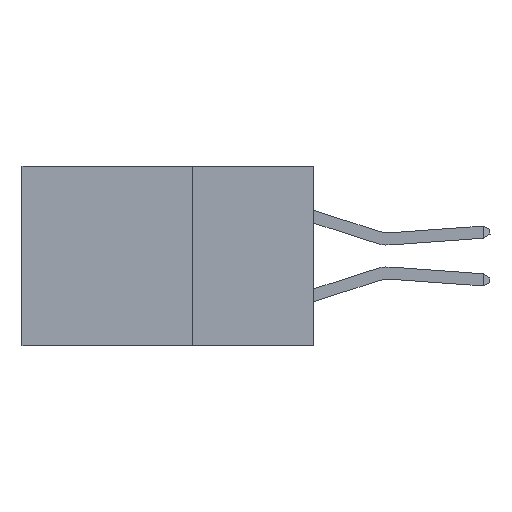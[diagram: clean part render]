
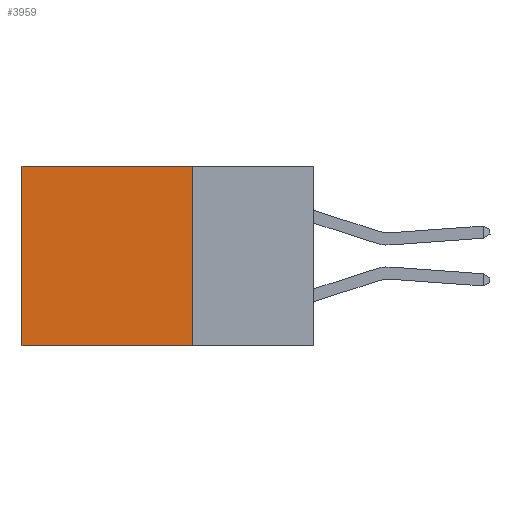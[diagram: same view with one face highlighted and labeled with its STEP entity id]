
A CAD part, left-side view. The second image highlights one B-rep face of the part: STEP entity #3959.
In plain terms, the highlighted planar face has unit normal (-1, 0, 0).
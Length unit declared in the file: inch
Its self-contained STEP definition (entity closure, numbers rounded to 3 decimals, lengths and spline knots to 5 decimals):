
#386 = CARTESIAN_POINT ( 'NONE',  ( 0.2875, 0.25, 0. ) ) ;
#739 = DIRECTION ( 'NONE',  ( 0., 1., 0. ) ) ;
#1558 = DIRECTION ( 'NONE',  ( 0., 0., -1. ) ) ;
#3090 = VECTOR ( 'NONE', #1558, 39.37008 ) ;
#3364 = PLANE ( 'NONE',  #15219 ) ;
#3959 = ADVANCED_FACE ( 'NONE', ( #17140 ), #3364, .F. ) ;
#4529 = CARTESIAN_POINT ( 'NONE',  ( 0.2875, 0.25, 0. ) ) ;
#6988 = ORIENTED_EDGE ( 'NONE', *, *, #11233, .T. ) ;
#7425 = CARTESIAN_POINT ( 'NONE',  ( 0.2875, 0.6, 0. ) ) ;
#7578 = LINE ( 'NONE', #13091, #13519 ) ;
#7761 = DIRECTION ( 'NONE',  ( 0., 0., -1. ) ) ;
#8370 = EDGE_LOOP ( 'NONE', ( #14749, #17801, #16557, #6988 ) ) ;
#8456 = LINE ( 'NONE', #4529, #12977 ) ;
#9046 = CARTESIAN_POINT ( 'NONE',  ( 0.2875, 0.25, -0.37 ) ) ;
#9297 = EDGE_CURVE ( 'NONE', #17252, #10705, #7578, .T. ) ;
#9495 = EDGE_CURVE ( 'NONE', #17716, #13127, #11349, .T. ) ;
#10125 = EDGE_CURVE ( 'NONE', #13127, #10705, #14400, .T. ) ;
#10705 = VERTEX_POINT ( 'NONE', #15139 ) ;
#11233 = EDGE_CURVE ( 'NONE', #17716, #17252, #8456, .T. ) ;
#11349 = LINE ( 'NONE', #14056, #3090 ) ;
#11608 = CARTESIAN_POINT ( 'NONE',  ( 0.2875, 0.25, -0.37 ) ) ;
#12096 = VECTOR ( 'NONE', #739, 39.37008 ) ;
#12977 = VECTOR ( 'NONE', #15205, 39.37008 ) ;
#13091 = CARTESIAN_POINT ( 'NONE',  ( 0.2875, 0.6, 0. ) ) ;
#13127 = VERTEX_POINT ( 'NONE', #9046 ) ;
#13519 = VECTOR ( 'NONE', #7761, 39.37008 ) ;
#14051 = DIRECTION ( 'NONE',  ( 0., 0., -1. ) ) ;
#14056 = CARTESIAN_POINT ( 'NONE',  ( 0.2875, 0.25, 0. ) ) ;
#14321 = DIRECTION ( 'NONE',  ( 1., 0., 0. ) ) ;
#14400 = LINE ( 'NONE', #11608, #12096 ) ;
#14749 = ORIENTED_EDGE ( 'NONE', *, *, #9297, .T. ) ;
#14881 = CARTESIAN_POINT ( 'NONE',  ( 0.2875, 0.25, 0. ) ) ;
#15139 = CARTESIAN_POINT ( 'NONE',  ( 0.2875, 0.6, -0.37 ) ) ;
#15205 = DIRECTION ( 'NONE',  ( 0., 1., 0. ) ) ;
#15219 = AXIS2_PLACEMENT_3D ( 'NONE', #386, #14321, #14051 ) ;
#16557 = ORIENTED_EDGE ( 'NONE', *, *, #9495, .F. ) ;
#17140 = FACE_OUTER_BOUND ( 'NONE', #8370, .T. ) ;
#17252 = VERTEX_POINT ( 'NONE', #7425 ) ;
#17716 = VERTEX_POINT ( 'NONE', #14881 ) ;
#17801 = ORIENTED_EDGE ( 'NONE', *, *, #10125, .F. ) ;
